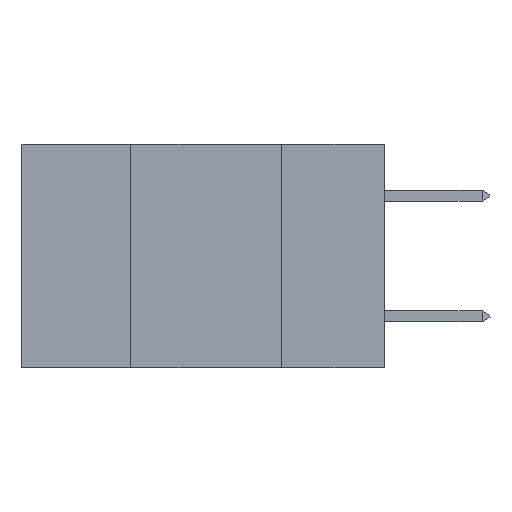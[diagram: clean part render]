
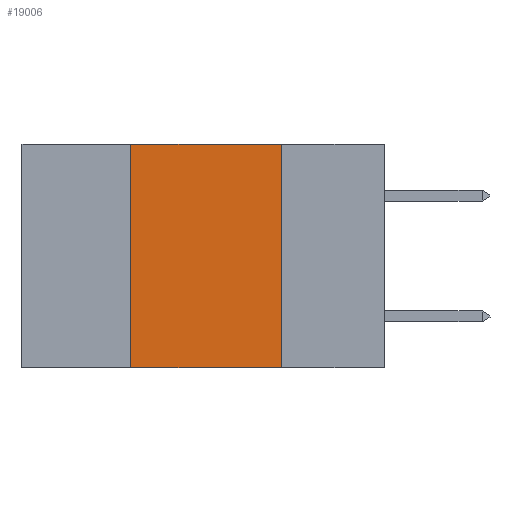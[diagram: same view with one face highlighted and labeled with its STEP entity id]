
A CAD part, left-side view. The second image highlights one B-rep face of the part: STEP entity #19006.
In plain terms, the highlighted planar face has unit normal (-1, 0, 0).
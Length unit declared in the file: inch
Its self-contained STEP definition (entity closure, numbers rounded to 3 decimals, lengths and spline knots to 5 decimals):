
#270 = VECTOR ( 'NONE', #1919, 39.37008 ) ;
#676 = PLANE ( 'NONE',  #13605 ) ;
#838 = LINE ( 'NONE', #15986, #270 ) ;
#1276 = LINE ( 'NONE', #12097, #18361 ) ;
#1919 = DIRECTION ( 'NONE',  ( 0., 0., 1. ) ) ;
#2195 = VERTEX_POINT ( 'NONE', #19853 ) ;
#2481 = DIRECTION ( 'NONE',  ( 0., 0., -1. ) ) ;
#2498 = ORIENTED_EDGE ( 'NONE', *, *, #16989, .F. ) ;
#2963 = CARTESIAN_POINT ( 'NONE',  ( 0., 0.42, 0. ) ) ;
#3140 = ORIENTED_EDGE ( 'NONE', *, *, #22135, .F. ) ;
#3255 = ORIENTED_EDGE ( 'NONE', *, *, #21309, .T. ) ;
#3261 = DIRECTION ( 'NONE',  ( 0., -1., 0. ) ) ;
#3347 = ORIENTED_EDGE ( 'NONE', *, *, #5787, .F. ) ;
#4183 = VERTEX_POINT ( 'NONE', #2963 ) ;
#4229 = CARTESIAN_POINT ( 'NONE',  ( 0., 0.6, 0. ) ) ;
#4850 = CARTESIAN_POINT ( 'NONE',  ( 0., 0.6, -0.37 ) ) ;
#5787 = EDGE_CURVE ( 'NONE', #4183, #2195, #1276, .T. ) ;
#6143 = CARTESIAN_POINT ( 'NONE',  ( 0., 0.42, -0.37 ) ) ;
#6494 = EDGE_LOOP ( 'NONE', ( #3140, #3347, #2498, #3255 ) ) ;
#6628 = VECTOR ( 'NONE', #6655, 39.37008 ) ;
#6655 = DIRECTION ( 'NONE',  ( 0., -1., 0. ) ) ;
#6867 = VERTEX_POINT ( 'NONE', #6143 ) ;
#7024 = FACE_OUTER_BOUND ( 'NONE', #6494, .T. ) ;
#7085 = CARTESIAN_POINT ( 'NONE',  ( 0., 0.17, -0.37 ) ) ;
#8693 = VERTEX_POINT ( 'NONE', #7085 ) ;
#9028 = DIRECTION ( 'NONE',  ( 0., 0., -1. ) ) ;
#10841 = CARTESIAN_POINT ( 'NONE',  ( 0., 0.17, 0. ) ) ;
#11853 = LINE ( 'NONE', #4850, #6628 ) ;
#12097 = CARTESIAN_POINT ( 'NONE',  ( 0., 0.6, 0. ) ) ;
#12351 = VECTOR ( 'NONE', #9028, 39.37008 ) ;
#13090 = DIRECTION ( 'NONE',  ( 1., 0., 0. ) ) ;
#13447 = LINE ( 'NONE', #10841, #12351 ) ;
#13605 = AXIS2_PLACEMENT_3D ( 'NONE', #4229, #13090, #2481 ) ;
#15986 = CARTESIAN_POINT ( 'NONE',  ( 0., 0.42, 0. ) ) ;
#16989 = EDGE_CURVE ( 'NONE', #6867, #4183, #838, .T. ) ;
#18361 = VECTOR ( 'NONE', #3261, 39.37008 ) ;
#19006 = ADVANCED_FACE ( 'NONE', ( #7024 ), #676, .F. ) ;
#19853 = CARTESIAN_POINT ( 'NONE',  ( 0., 0.17, 0. ) ) ;
#21309 = EDGE_CURVE ( 'NONE', #6867, #8693, #11853, .T. ) ;
#22135 = EDGE_CURVE ( 'NONE', #2195, #8693, #13447, .T. ) ;
